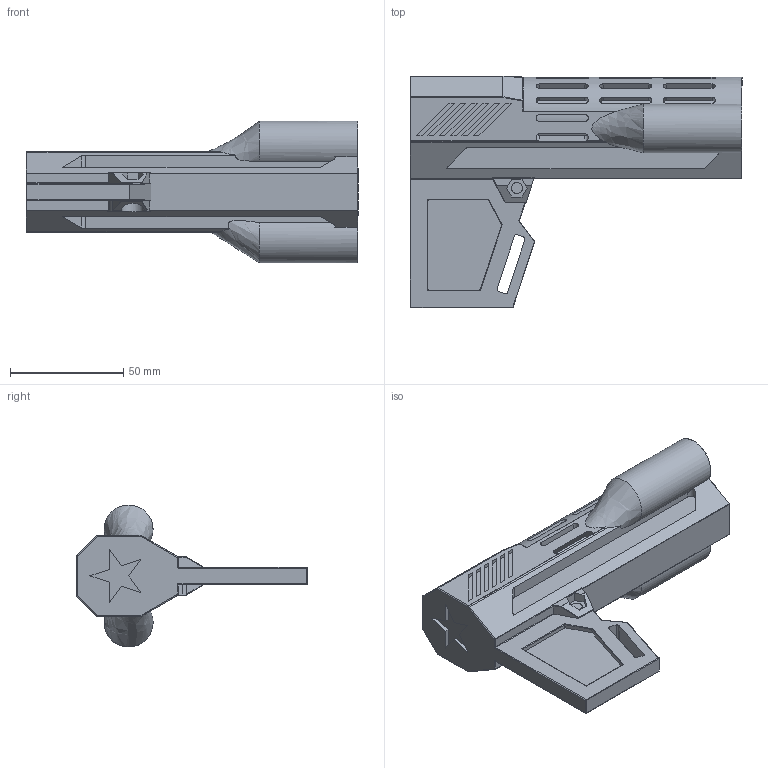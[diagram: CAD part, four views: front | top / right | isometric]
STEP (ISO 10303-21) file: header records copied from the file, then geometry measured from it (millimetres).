
FILE_DESCRIPTION(/* description */ ('STEP AP214'),/* implementation_level */ '2;1');
FILE_NAME(/* author */ (''),/* organization */ (''),/* preprocessor_version */ 'ST-DEVELOPER v18.1',/* originating_system */ ' ',/* authorisation */ ' ');
FILE_SCHEMA (('AUTOMOTIVE_DESIGN {1 0 10303 214 3 1 1}'));
Length unit declared in the file: metre
Products named in the file (1): Part 1
Bounding box: 146.33 x 102 x 62.58 mm (x, y, z)
Volume: 223390.7 mm3; surface area: 39786.9 mm2
Topology: 1 solids, 11 shells, 603 faces, 1561 edges, 1005 vertices
Faces by surface type: plane 288, cylinder 178, bspline 122, torus 14, sphere 1
Full cylindrical faces by diameter (mm): 4.915 x2, 4.996 x1, 5.003 x1, 9.831 x1
Entity records: 21847 total; most frequent: CARTESIAN_POINT 7838, ORIENTED_EDGE 3074, DIRECTION 2250, EDGE_CURVE 1537, VERTEX_POINT 1002, LINE 900, VECTOR 900, AXIS2_PLACEMENT_3D 675
